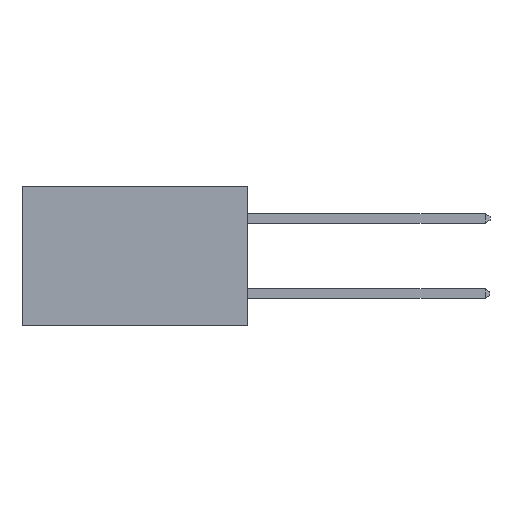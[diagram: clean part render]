
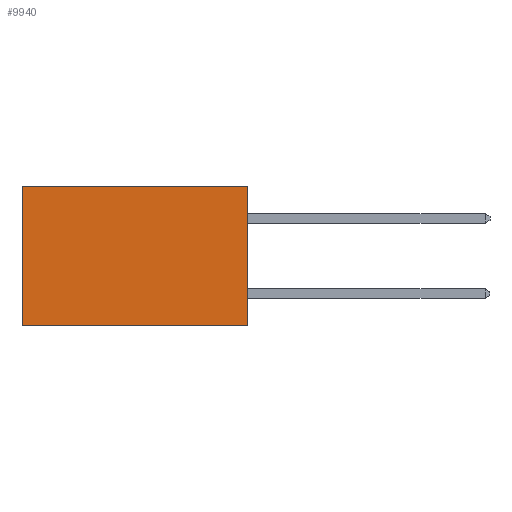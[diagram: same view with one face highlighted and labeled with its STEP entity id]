
A CAD part, left-side view. The second image highlights one B-rep face of the part: STEP entity #9940.
In plain terms, the highlighted planar face has unit normal (-1, 0, 0).
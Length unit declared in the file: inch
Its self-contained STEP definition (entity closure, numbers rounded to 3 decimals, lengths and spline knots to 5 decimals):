
#188 = CARTESIAN_POINT ( 'NONE',  ( 0.298, 0., 0. ) ) ;
#339 = ORIENTED_EDGE ( 'NONE', *, *, #9715, .F. ) ;
#504 = LINE ( 'NONE', #5893, #829 ) ;
#764 = VECTOR ( 'NONE', #1058, 39.37008 ) ;
#829 = VECTOR ( 'NONE', #5966, 39.37008 ) ;
#936 = CARTESIAN_POINT ( 'NONE',  ( 0.298, 0., 0. ) ) ;
#1058 = DIRECTION ( 'NONE',  ( 0., 1., 0. ) ) ;
#1086 = CARTESIAN_POINT ( 'NONE',  ( 0.298, 0., -0.37 ) ) ;
#1250 = VERTEX_POINT ( 'NONE', #1913 ) ;
#1913 = CARTESIAN_POINT ( 'NONE',  ( 0.298, 0.6, 0. ) ) ;
#2537 = LINE ( 'NONE', #936, #13333 ) ;
#3568 = LINE ( 'NONE', #1086, #764 ) ;
#3973 = ORIENTED_EDGE ( 'NONE', *, *, #13261, .F. ) ;
#4908 = VERTEX_POINT ( 'NONE', #188 ) ;
#5028 = CARTESIAN_POINT ( 'NONE',  ( 0.298, 0.6, -0.37 ) ) ;
#5207 = AXIS2_PLACEMENT_3D ( 'NONE', #11682, #5444, #12704 ) ;
#5444 = DIRECTION ( 'NONE',  ( 1., 0., 0. ) ) ;
#5893 = CARTESIAN_POINT ( 'NONE',  ( 0.298, 0., 0. ) ) ;
#5966 = DIRECTION ( 'NONE',  ( 0., 1., 0. ) ) ;
#6278 = ORIENTED_EDGE ( 'NONE', *, *, #7326, .T. ) ;
#6852 = EDGE_LOOP ( 'NONE', ( #6278, #339, #3973, #11509 ) ) ;
#7326 = EDGE_CURVE ( 'NONE', #1250, #12242, #12829, .T. ) ;
#7658 = EDGE_CURVE ( 'NONE', #4908, #1250, #504, .T. ) ;
#8512 = DIRECTION ( 'NONE',  ( 0., 0., -1. ) ) ;
#8559 = CARTESIAN_POINT ( 'NONE',  ( 0.298, 0.6, 0. ) ) ;
#8628 = CARTESIAN_POINT ( 'NONE',  ( 0.298, 0., -0.37 ) ) ;
#8941 = VERTEX_POINT ( 'NONE', #8628 ) ;
#9373 = DIRECTION ( 'NONE',  ( 0., 0., -1. ) ) ;
#9581 = PLANE ( 'NONE',  #5207 ) ;
#9715 = EDGE_CURVE ( 'NONE', #8941, #12242, #3568, .T. ) ;
#9940 = ADVANCED_FACE ( 'NONE', ( #11470 ), #9581, .F. ) ;
#11470 = FACE_OUTER_BOUND ( 'NONE', #6852, .T. ) ;
#11509 = ORIENTED_EDGE ( 'NONE', *, *, #7658, .T. ) ;
#11682 = CARTESIAN_POINT ( 'NONE',  ( 0.298, 0., 0. ) ) ;
#12242 = VERTEX_POINT ( 'NONE', #5028 ) ;
#12487 = VECTOR ( 'NONE', #8512, 39.37008 ) ;
#12704 = DIRECTION ( 'NONE',  ( 0., 0., -1. ) ) ;
#12829 = LINE ( 'NONE', #8559, #12487 ) ;
#13261 = EDGE_CURVE ( 'NONE', #4908, #8941, #2537, .T. ) ;
#13333 = VECTOR ( 'NONE', #9373, 39.37008 ) ;
